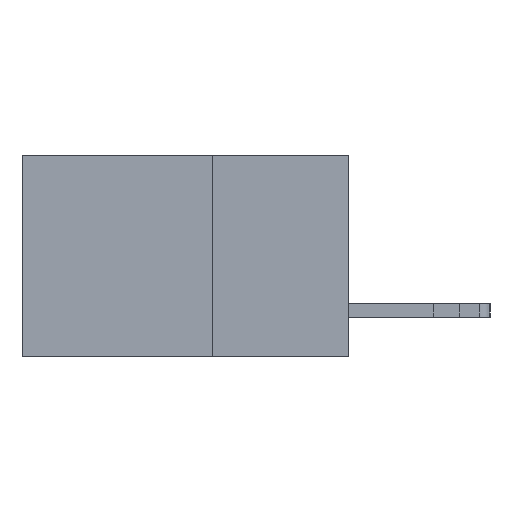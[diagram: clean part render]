
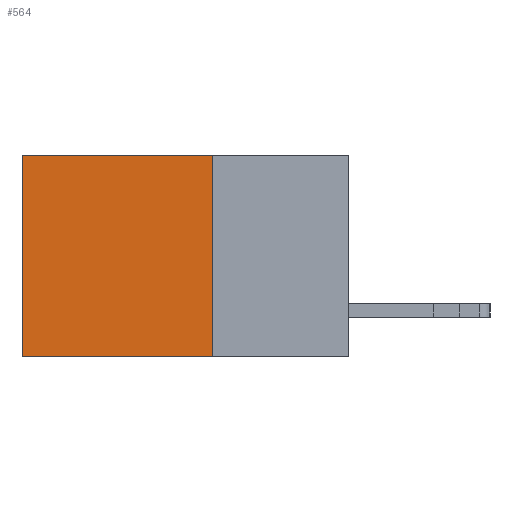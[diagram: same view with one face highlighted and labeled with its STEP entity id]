
A CAD part, left-side view. The second image highlights one B-rep face of the part: STEP entity #564.
In plain terms, the highlighted planar face has unit normal (-1, 0, 0).
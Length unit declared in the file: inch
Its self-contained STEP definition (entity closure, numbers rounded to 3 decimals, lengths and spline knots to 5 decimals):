
#396 = VECTOR ( 'NONE', #4118, 39.37008 ) ;
#538 = ORIENTED_EDGE ( 'NONE', *, *, #9224, .F. ) ;
#564 = ADVANCED_FACE ( 'NONE', ( #2984 ), #8586, .F. ) ;
#886 = VERTEX_POINT ( 'NONE', #5845 ) ;
#975 = LINE ( 'NONE', #1451, #396 ) ;
#1371 = DIRECTION ( 'NONE',  ( 0., 0., -1. ) ) ;
#1382 = LINE ( 'NONE', #6578, #3713 ) ;
#1451 = CARTESIAN_POINT ( 'NONE',  ( 0.2615, 0.6, -0.37 ) ) ;
#1725 = EDGE_LOOP ( 'NONE', ( #8242, #538, #2889, #8697 ) ) ;
#2066 = CARTESIAN_POINT ( 'NONE',  ( 0.2615, 0.25, 0. ) ) ;
#2229 = VERTEX_POINT ( 'NONE', #9147 ) ;
#2774 = VECTOR ( 'NONE', #7908, 39.37008 ) ;
#2889 = ORIENTED_EDGE ( 'NONE', *, *, #10215, .F. ) ;
#2984 = FACE_OUTER_BOUND ( 'NONE', #1725, .T. ) ;
#3050 = AXIS2_PLACEMENT_3D ( 'NONE', #9697, #10408, #1371 ) ;
#3713 = VECTOR ( 'NONE', #4917, 39.37008 ) ;
#4118 = DIRECTION ( 'NONE',  ( 0., 0., -1. ) ) ;
#4403 = DIRECTION ( 'NONE',  ( 0., 1., 0. ) ) ;
#4905 = VECTOR ( 'NONE', #4403, 39.37008 ) ;
#4917 = DIRECTION ( 'NONE',  ( 0., 0., -1. ) ) ;
#5337 = CARTESIAN_POINT ( 'NONE',  ( 0.2615, 0.6, -0.37 ) ) ;
#5845 = CARTESIAN_POINT ( 'NONE',  ( 0.2615, 0.6, 0. ) ) ;
#6578 = CARTESIAN_POINT ( 'NONE',  ( 0.2615, 0.25, -0.37 ) ) ;
#6869 = CARTESIAN_POINT ( 'NONE',  ( 0.2615, 0.25, -0.37 ) ) ;
#7046 = VERTEX_POINT ( 'NONE', #7832 ) ;
#7347 = LINE ( 'NONE', #6869, #4905 ) ;
#7466 = VERTEX_POINT ( 'NONE', #5337 ) ;
#7832 = CARTESIAN_POINT ( 'NONE',  ( 0.2615, 0.25, -0.37 ) ) ;
#7908 = DIRECTION ( 'NONE',  ( 0., 1., 0. ) ) ;
#8196 = EDGE_CURVE ( 'NONE', #2229, #886, #9020, .T. ) ;
#8242 = ORIENTED_EDGE ( 'NONE', *, *, #9011, .T. ) ;
#8586 = PLANE ( 'NONE',  #3050 ) ;
#8697 = ORIENTED_EDGE ( 'NONE', *, *, #8196, .T. ) ;
#9011 = EDGE_CURVE ( 'NONE', #886, #7466, #975, .T. ) ;
#9020 = LINE ( 'NONE', #2066, #2774 ) ;
#9147 = CARTESIAN_POINT ( 'NONE',  ( 0.2615, 0.25, 0. ) ) ;
#9224 = EDGE_CURVE ( 'NONE', #7046, #7466, #7347, .T. ) ;
#9697 = CARTESIAN_POINT ( 'NONE',  ( 0.2615, 0.25, -0.37 ) ) ;
#10215 = EDGE_CURVE ( 'NONE', #2229, #7046, #1382, .T. ) ;
#10408 = DIRECTION ( 'NONE',  ( 1., 0., 0. ) ) ;
